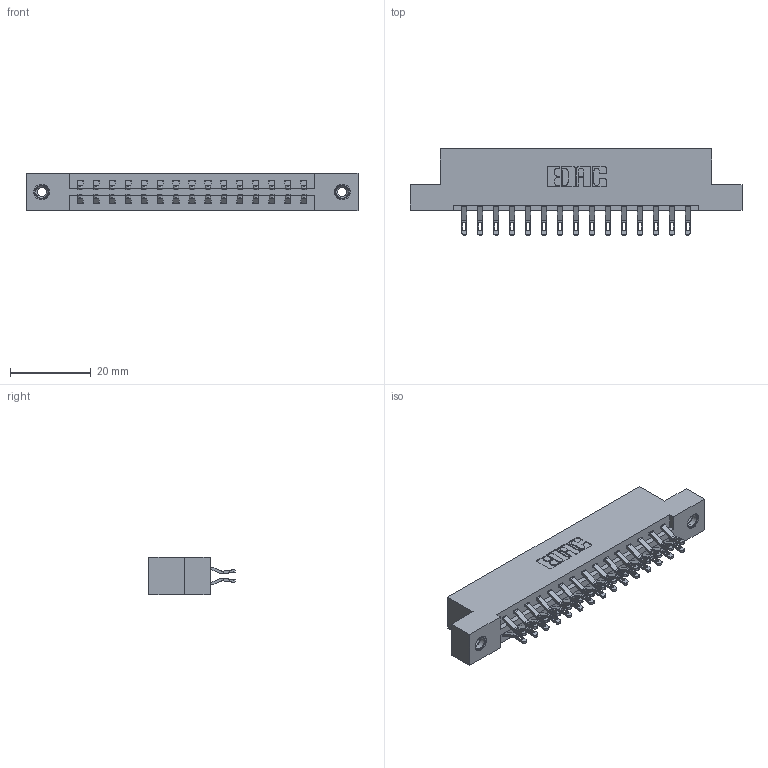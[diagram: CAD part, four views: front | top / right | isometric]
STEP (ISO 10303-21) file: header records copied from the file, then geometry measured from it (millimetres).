
FILE_DESCRIPTION (( 'STEP AP203' ), '1' );
FILE_NAME ('337-030-555-208.STEP', '2019-10-08T18:54:13', ( '' ), ( '' ), 'SwSTEP 2.0', 'SolidWorks 2016', '' );
FILE_SCHEMA (( 'CONFIG_CONTROL_DESIGN' ));
Length unit declared in the file: inch
Products named in the file (4): 337 Part_Flush Mounting Lugs - 0.156 Dia-TI; 345-292-001_555 Tail; 345-250-001_345-250-003-102; 337-030-555-208
Assembly tree (33 placements, depth 2):
  337-030-555-208
    337 Part_Flush Mounting Lugs - 0.156 Dia-TI
    345-292-001_555 Tail  x30
    345-250-001_345-250-003-102  x2
Bounding box: 82.45 x 21.47 x 9.4 mm (x, y, z)
Volume: 8410.2 mm3; surface area: 9597.3 mm2
Topology: 33 solids, 33 shells, 1974 faces, 6117 edges, 4070 vertices
Faces by surface type: plane 1182, cylinder 776, cone 12, torus 4
Entity records: 16634 total; most frequent: CARTESIAN_POINT 2839, ORIENTED_EDGE 2738, DIRECTION 2467, EDGE_CURVE 1369, LINE 1201, VECTOR 1201, VERTEX_POINT 908, AXIS2_PLACEMENT_3D 633
